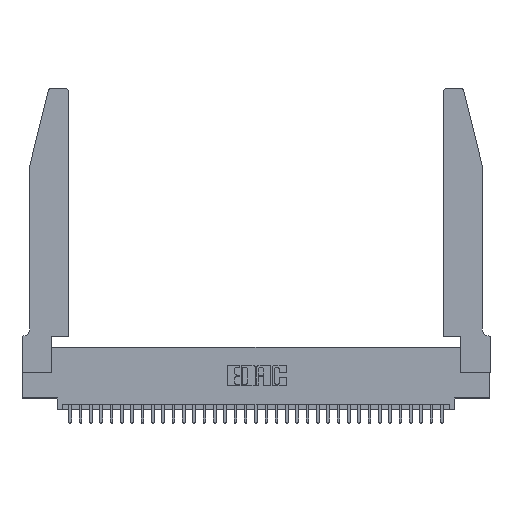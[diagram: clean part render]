
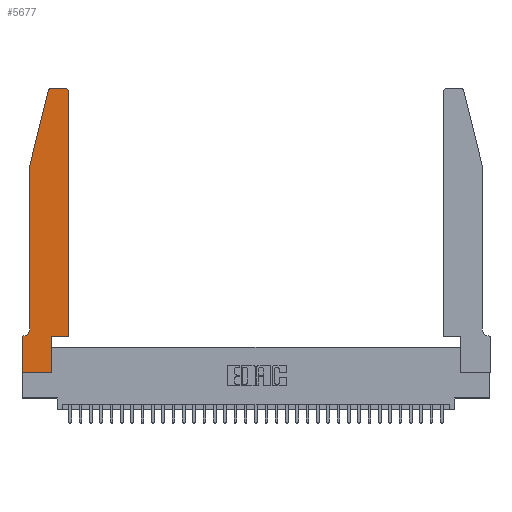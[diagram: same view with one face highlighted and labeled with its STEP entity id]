
A CAD part, top view. The second image highlights one B-rep face of the part: STEP entity #5677.
In plain terms, the highlighted planar face has unit normal (0, 0, 1).
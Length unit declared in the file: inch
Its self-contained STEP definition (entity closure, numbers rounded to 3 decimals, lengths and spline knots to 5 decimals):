
#290 = VECTOR ( 'NONE', #4223, 39.37008 ) ;
#802 = ORIENTED_EDGE ( 'NONE', *, *, #3869, .T. ) ;
#1048 = CIRCLE ( 'NONE', #10662, 0.03 ) ;
#1844 = EDGE_CURVE ( 'NONE', #10753, #19277, #29808, .T. ) ;
#1882 = VECTOR ( 'NONE', #21091, 39.37008 ) ;
#1947 = LINE ( 'NONE', #20837, #23246 ) ;
#2073 = CARTESIAN_POINT ( 'NONE',  ( 0.2605, 2.75, 0.37 ) ) ;
#2137 = ORIENTED_EDGE ( 'NONE', *, *, #1844, .T. ) ;
#2240 = VERTEX_POINT ( 'NONE', #17276 ) ;
#2523 = CARTESIAN_POINT ( 'NONE',  ( 0.4505, 2.72, 0.37 ) ) ;
#3606 = CARTESIAN_POINT ( 'NONE',  ( 0.0755, 0.42, 0.37 ) ) ;
#3869 = EDGE_CURVE ( 'NONE', #19277, #5399, #11213, .T. ) ;
#4223 = DIRECTION ( 'NONE',  ( -0.239, -0.971, 0. ) ) ;
#4637 = CARTESIAN_POINT ( 'NONE',  ( 0.0755, 2., 0.37 ) ) ;
#4761 = CARTESIAN_POINT ( 'NONE',  ( 0., 0., 0.37 ) ) ;
#4926 = CARTESIAN_POINT ( 'NONE',  ( 0.4205, 2.75, 0.37 ) ) ;
#5116 = ORIENTED_EDGE ( 'NONE', *, *, #12695, .T. ) ;
#5270 = LINE ( 'NONE', #4637, #22369 ) ;
#5399 = VERTEX_POINT ( 'NONE', #2523 ) ;
#5677 = ADVANCED_FACE ( 'NONE', ( #16999 ), #6868, .T. ) ;
#6446 = CARTESIAN_POINT ( 'NONE',  ( 0.4505, 0.35, 0.37 ) ) ;
#6771 = DIRECTION ( 'NONE',  ( 1., 0., 0. ) ) ;
#6868 = PLANE ( 'NONE',  #24051 ) ;
#6996 = DIRECTION ( 'NONE',  ( 0., 0., 1. ) ) ;
#7208 = ORIENTED_EDGE ( 'NONE', *, *, #8614, .T. ) ;
#7236 = VECTOR ( 'NONE', #19125, 39.37008 ) ;
#7644 = VERTEX_POINT ( 'NONE', #22519 ) ;
#7700 = VERTEX_POINT ( 'NONE', #14419 ) ;
#8116 = LINE ( 'NONE', #2073, #1882 ) ;
#8439 = ORIENTED_EDGE ( 'NONE', *, *, #29401, .T. ) ;
#8577 = ORIENTED_EDGE ( 'NONE', *, *, #13838, .T. ) ;
#8614 = EDGE_CURVE ( 'NONE', #5399, #10884, #1048, .T. ) ;
#8872 = DIRECTION ( 'NONE',  ( -1., 0., 0. ) ) ;
#8891 = VERTEX_POINT ( 'NONE', #9282 ) ;
#9282 = CARTESIAN_POINT ( 'NONE',  ( 0.25487, 2.72718, 0.37 ) ) ;
#9703 = CARTESIAN_POINT ( 'NONE',  ( 0.0755, 0.35, 0.37 ) ) ;
#9919 = EDGE_CURVE ( 'NONE', #24963, #21688, #28233, .T. ) ;
#10355 = DIRECTION ( 'NONE',  ( 0., -1., 0. ) ) ;
#10537 = CIRCLE ( 'NONE', #11585, 0.03 ) ;
#10662 = AXIS2_PLACEMENT_3D ( 'NONE', #13715, #27341, #6771 ) ;
#10753 = VERTEX_POINT ( 'NONE', #28702 ) ;
#10884 = VERTEX_POINT ( 'NONE', #4926 ) ;
#11213 = LINE ( 'NONE', #16144, #23841 ) ;
#11398 = DIRECTION ( 'NONE',  ( 0., 0., -1. ) ) ;
#11585 = AXIS2_PLACEMENT_3D ( 'NONE', #18972, #27393, #24676 ) ;
#11803 = AXIS2_PLACEMENT_3D ( 'NONE', #14319, #11398, #8872 ) ;
#12615 = ORIENTED_EDGE ( 'NONE', *, *, #18600, .T. ) ;
#12695 = EDGE_CURVE ( 'NONE', #10884, #7644, #8116, .T. ) ;
#13715 = CARTESIAN_POINT ( 'NONE',  ( 0.4205, 2.72, 0.37 ) ) ;
#13838 = EDGE_CURVE ( 'NONE', #7644, #8891, #10537, .T. ) ;
#14319 = CARTESIAN_POINT ( 'NONE',  ( 0.0055, 0.42, 0.37 ) ) ;
#14419 = CARTESIAN_POINT ( 'NONE',  ( 0.0055, 0.35, 0.37 ) ) ;
#15277 = DIRECTION ( 'NONE',  ( 1., 0., 0. ) ) ;
#16079 = LINE ( 'NONE', #23370, #29499 ) ;
#16144 = CARTESIAN_POINT ( 'NONE',  ( 0.4505, 0.35, 0.37 ) ) ;
#16563 = LINE ( 'NONE', #9703, #26663 ) ;
#16999 = FACE_OUTER_BOUND ( 'NONE', #26124, .T. ) ;
#17276 = CARTESIAN_POINT ( 'NONE',  ( 0.0755, 2., 0.37 ) ) ;
#17311 = CARTESIAN_POINT ( 'NONE',  ( 0.0755, 2., 0.37 ) ) ;
#17548 = EDGE_CURVE ( 'NONE', #7700, #24963, #16563, .T. ) ;
#17676 = ORIENTED_EDGE ( 'NONE', *, *, #31018, .T. ) ;
#17748 = ORIENTED_EDGE ( 'NONE', *, *, #17548, .T. ) ;
#17870 = DIRECTION ( 'NONE',  ( 0., -1., 0. ) ) ;
#18600 = EDGE_CURVE ( 'NONE', #2240, #18632, #5270, .T. ) ;
#18632 = VERTEX_POINT ( 'NONE', #3606 ) ;
#18972 = CARTESIAN_POINT ( 'NONE',  ( 0.284, 2.72, 0.37 ) ) ;
#19125 = DIRECTION ( 'NONE',  ( 1., 0., 0. ) ) ;
#19277 = VERTEX_POINT ( 'NONE', #6446 ) ;
#19679 = CARTESIAN_POINT ( 'NONE',  ( 0., 0.35, 0.37 ) ) ;
#19813 = VECTOR ( 'NONE', #10355, 39.37008 ) ;
#20837 = CARTESIAN_POINT ( 'NONE',  ( 0.2865, 0.35, 0.37 ) ) ;
#21091 = DIRECTION ( 'NONE',  ( -1., 0., 0. ) ) ;
#21688 = VERTEX_POINT ( 'NONE', #4761 ) ;
#22032 = CARTESIAN_POINT ( 'NONE',  ( 0.4505, 0.35, 0.37 ) ) ;
#22369 = VECTOR ( 'NONE', #17870, 39.37008 ) ;
#22519 = CARTESIAN_POINT ( 'NONE',  ( 0.284, 2.75, 0.37 ) ) ;
#23246 = VECTOR ( 'NONE', #29047, 39.37008 ) ;
#23370 = CARTESIAN_POINT ( 'NONE',  ( 0., 0., 0.37 ) ) ;
#23841 = VECTOR ( 'NONE', #31416, 39.37008 ) ;
#23976 = DIRECTION ( 'NONE',  ( 1., 0., 0. ) ) ;
#24051 = AXIS2_PLACEMENT_3D ( 'NONE', #19679, #6996, #23976 ) ;
#24615 = EDGE_CURVE ( 'NONE', #18632, #7700, #24635, .T. ) ;
#24635 = CIRCLE ( 'NONE', #11803, 0.07 ) ;
#24676 = DIRECTION ( 'NONE',  ( 1., 0., 0. ) ) ;
#24963 = VERTEX_POINT ( 'NONE', #29356 ) ;
#26124 = EDGE_LOOP ( 'NONE', ( #5116, #8577, #29936, #12615, #28032, #17748, #27727, #17676, #8439, #2137, #802, #7208 ) ) ;
#26302 = LINE ( 'NONE', #17311, #290 ) ;
#26663 = VECTOR ( 'NONE', #31273, 39.37008 ) ;
#26880 = CARTESIAN_POINT ( 'NONE',  ( 0.2865, 0., 0.37 ) ) ;
#27341 = DIRECTION ( 'NONE',  ( 0., 0., 1. ) ) ;
#27393 = DIRECTION ( 'NONE',  ( 0., 0., 1. ) ) ;
#27727 = ORIENTED_EDGE ( 'NONE', *, *, #9919, .T. ) ;
#28032 = ORIENTED_EDGE ( 'NONE', *, *, #24615, .T. ) ;
#28233 = LINE ( 'NONE', #29098, #19813 ) ;
#28702 = CARTESIAN_POINT ( 'NONE',  ( 0.2865, 0.35, 0.37 ) ) ;
#29047 = DIRECTION ( 'NONE',  ( 0., 1., 0. ) ) ;
#29098 = CARTESIAN_POINT ( 'NONE',  ( 0., 0., 0.37 ) ) ;
#29356 = CARTESIAN_POINT ( 'NONE',  ( 0., 0.35, 0.37 ) ) ;
#29401 = EDGE_CURVE ( 'NONE', #33671, #10753, #1947, .T. ) ;
#29499 = VECTOR ( 'NONE', #15277, 39.37008 ) ;
#29808 = LINE ( 'NONE', #22032, #7236 ) ;
#29936 = ORIENTED_EDGE ( 'NONE', *, *, #33307, .T. ) ;
#31018 = EDGE_CURVE ( 'NONE', #21688, #33671, #16079, .T. ) ;
#31273 = DIRECTION ( 'NONE',  ( -1., 0., 0. ) ) ;
#31416 = DIRECTION ( 'NONE',  ( 0., 1., 0. ) ) ;
#33307 = EDGE_CURVE ( 'NONE', #8891, #2240, #26302, .T. ) ;
#33671 = VERTEX_POINT ( 'NONE', #26880 ) ;
